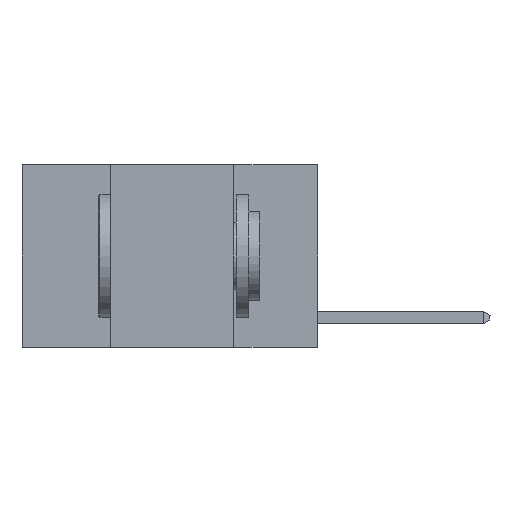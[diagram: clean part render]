
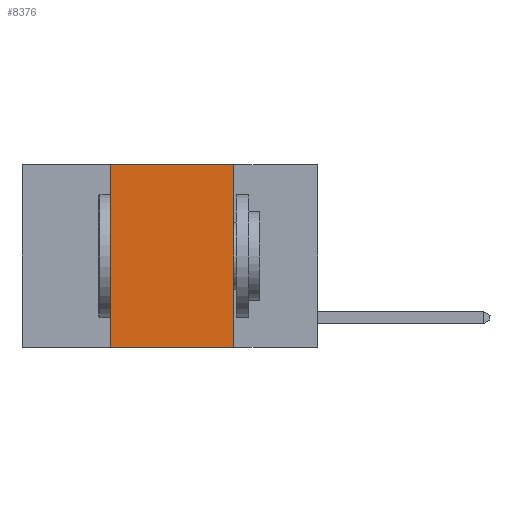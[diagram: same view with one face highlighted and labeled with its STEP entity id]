
A CAD part, left-side view. The second image highlights one B-rep face of the part: STEP entity #8376.
In plain terms, the highlighted planar face has unit normal (-1, 0, 0).
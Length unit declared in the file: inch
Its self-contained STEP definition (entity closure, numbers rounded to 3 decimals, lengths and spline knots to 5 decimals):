
#227 = DIRECTION ( 'NONE',  ( 0., 0., -1. ) ) ;
#727 = CARTESIAN_POINT ( 'NONE',  ( 0., 0.6, 0. ) ) ;
#1046 = ORIENTED_EDGE ( 'NONE', *, *, #9276, .T. ) ;
#1074 = ORIENTED_EDGE ( 'NONE', *, *, #2511, .F. ) ;
#1262 = VECTOR ( 'NONE', #10655, 39.37008 ) ;
#1328 = DIRECTION ( 'NONE',  ( 0., 0., 1. ) ) ;
#1729 = VERTEX_POINT ( 'NONE', #6568 ) ;
#2143 = CARTESIAN_POINT ( 'NONE',  ( 0., 0.6, 0. ) ) ;
#2193 = FACE_OUTER_BOUND ( 'NONE', #6384, .T. ) ;
#2511 = EDGE_CURVE ( 'NONE', #1729, #6807, #8884, .T. ) ;
#2617 = AXIS2_PLACEMENT_3D ( 'NONE', #2143, #8588, #4892 ) ;
#3140 = LINE ( 'NONE', #9405, #3696 ) ;
#3562 = ORIENTED_EDGE ( 'NONE', *, *, #10339, .F. ) ;
#3696 = VECTOR ( 'NONE', #227, 39.37008 ) ;
#3960 = LINE ( 'NONE', #5982, #5760 ) ;
#4248 = LINE ( 'NONE', #9609, #1262 ) ;
#4892 = DIRECTION ( 'NONE',  ( 0., 0., -1. ) ) ;
#5760 = VECTOR ( 'NONE', #1328, 39.37008 ) ;
#5878 = CARTESIAN_POINT ( 'NONE',  ( 0., 0.17, -0.37 ) ) ;
#5982 = CARTESIAN_POINT ( 'NONE',  ( 0., 0.42, 0. ) ) ;
#6384 = EDGE_LOOP ( 'NONE', ( #10962, #1074, #3562, #1046 ) ) ;
#6568 = CARTESIAN_POINT ( 'NONE',  ( 0., 0.42, 0. ) ) ;
#6807 = VERTEX_POINT ( 'NONE', #10837 ) ;
#7091 = DIRECTION ( 'NONE',  ( 0., -1., 0. ) ) ;
#7369 = EDGE_CURVE ( 'NONE', #6807, #8652, #3140, .T. ) ;
#7955 = VECTOR ( 'NONE', #7091, 39.37008 ) ;
#8344 = PLANE ( 'NONE',  #2617 ) ;
#8376 = ADVANCED_FACE ( 'NONE', ( #2193 ), #8344, .F. ) ;
#8588 = DIRECTION ( 'NONE',  ( 1., 0., 0. ) ) ;
#8652 = VERTEX_POINT ( 'NONE', #5878 ) ;
#8884 = LINE ( 'NONE', #727, #7955 ) ;
#9144 = VERTEX_POINT ( 'NONE', #9556 ) ;
#9276 = EDGE_CURVE ( 'NONE', #9144, #8652, #4248, .T. ) ;
#9405 = CARTESIAN_POINT ( 'NONE',  ( 0., 0.17, 0. ) ) ;
#9556 = CARTESIAN_POINT ( 'NONE',  ( 0., 0.42, -0.37 ) ) ;
#9609 = CARTESIAN_POINT ( 'NONE',  ( 0., 0.6, -0.37 ) ) ;
#10339 = EDGE_CURVE ( 'NONE', #9144, #1729, #3960, .T. ) ;
#10655 = DIRECTION ( 'NONE',  ( 0., -1., 0. ) ) ;
#10837 = CARTESIAN_POINT ( 'NONE',  ( 0., 0.17, 0. ) ) ;
#10962 = ORIENTED_EDGE ( 'NONE', *, *, #7369, .F. ) ;
